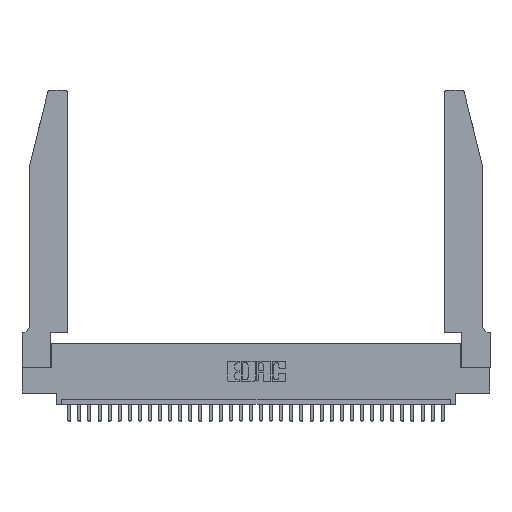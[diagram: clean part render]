
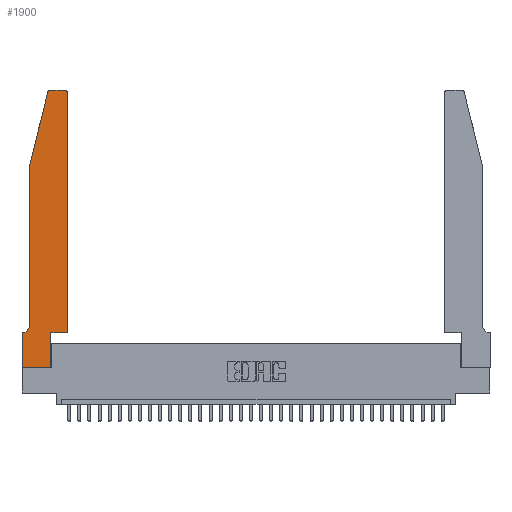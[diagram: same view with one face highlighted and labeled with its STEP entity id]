
A CAD part, top view. The second image highlights one B-rep face of the part: STEP entity #1900.
In plain terms, the highlighted planar face has unit normal (0, 0, 1).
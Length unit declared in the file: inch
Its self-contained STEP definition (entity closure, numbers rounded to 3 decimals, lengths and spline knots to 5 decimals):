
#378 = EDGE_CURVE ( 'NONE', #31666, #30595, #3601, .T. ) ;
#894 = CARTESIAN_POINT ( 'NONE',  ( 0.0055, 0.42, 0.37 ) ) ;
#1523 = VECTOR ( 'NONE', #24377, 39.37008 ) ;
#1820 = ORIENTED_EDGE ( 'NONE', *, *, #32897, .T. ) ;
#1900 = ADVANCED_FACE ( 'NONE', ( #3408 ), #12064, .T. ) ;
#1979 = CARTESIAN_POINT ( 'NONE',  ( 0.4205, 2.75, 0.37 ) ) ;
#1986 = LINE ( 'NONE', #2097, #11055 ) ;
#2097 = CARTESIAN_POINT ( 'NONE',  ( 0.2605, 2.75, 0.37 ) ) ;
#2234 = DIRECTION ( 'NONE',  ( 0., -1., 0. ) ) ;
#2243 = AXIS2_PLACEMENT_3D ( 'NONE', #894, #24611, #29582 ) ;
#2337 = VERTEX_POINT ( 'NONE', #3133 ) ;
#2358 = CARTESIAN_POINT ( 'NONE',  ( 0., 0.35, 0.37 ) ) ;
#2550 = DIRECTION ( 'NONE',  ( -1., 0., 0. ) ) ;
#2717 = ORIENTED_EDGE ( 'NONE', *, *, #17751, .T. ) ;
#3133 = CARTESIAN_POINT ( 'NONE',  ( 0.0755, 0.42, 0.37 ) ) ;
#3337 = CARTESIAN_POINT ( 'NONE',  ( 0.4505, 0.35, 0.37 ) ) ;
#3408 = FACE_OUTER_BOUND ( 'NONE', #11539, .T. ) ;
#3601 = LINE ( 'NONE', #29055, #6927 ) ;
#3641 = CARTESIAN_POINT ( 'NONE',  ( 0.0755, 2., 0.37 ) ) ;
#4012 = CARTESIAN_POINT ( 'NONE',  ( 0.284, 2.75, 0.37 ) ) ;
#4255 = CARTESIAN_POINT ( 'NONE',  ( 0.2865, 0., 0.37 ) ) ;
#4314 = DIRECTION ( 'NONE',  ( 0., 0., 1. ) ) ;
#4411 = CARTESIAN_POINT ( 'NONE',  ( 0., 0., 0.37 ) ) ;
#4863 = ORIENTED_EDGE ( 'NONE', *, *, #7968, .T. ) ;
#4931 = DIRECTION ( 'NONE',  ( 0., 1., 0. ) ) ;
#5988 = DIRECTION ( 'NONE',  ( 1., 0., 0. ) ) ;
#5998 = DIRECTION ( 'NONE',  ( 0., 1., 0. ) ) ;
#6377 = CIRCLE ( 'NONE', #2243, 0.07 ) ;
#6534 = EDGE_CURVE ( 'NONE', #27630, #6646, #17616, .T. ) ;
#6646 = VERTEX_POINT ( 'NONE', #3641 ) ;
#6927 = VECTOR ( 'NONE', #29381, 39.37008 ) ;
#6980 = ORIENTED_EDGE ( 'NONE', *, *, #10887, .T. ) ;
#7105 = VERTEX_POINT ( 'NONE', #20014 ) ;
#7160 = CARTESIAN_POINT ( 'NONE',  ( 0.25487, 2.72718, 0.37 ) ) ;
#7968 = EDGE_CURVE ( 'NONE', #30595, #17654, #28152, .T. ) ;
#8931 = LINE ( 'NONE', #17839, #16777 ) ;
#8942 = CIRCLE ( 'NONE', #20503, 0.03 ) ;
#9173 = EDGE_CURVE ( 'NONE', #28556, #18429, #1986, .T. ) ;
#9708 = VERTEX_POINT ( 'NONE', #11129 ) ;
#10887 = EDGE_CURVE ( 'NONE', #28252, #9708, #18419, .T. ) ;
#11055 = VECTOR ( 'NONE', #2550, 39.37008 ) ;
#11129 = CARTESIAN_POINT ( 'NONE',  ( 0.4505, 2.72, 0.37 ) ) ;
#11187 = CARTESIAN_POINT ( 'NONE',  ( 0., 0., 0.37 ) ) ;
#11539 = EDGE_LOOP ( 'NONE', ( #31238, #1820, #30203, #26848, #13171, #14129, #4863, #19136, #22132, #2717, #6980, #32469 ) ) ;
#11841 = VECTOR ( 'NONE', #16122, 39.37008 ) ;
#12064 = PLANE ( 'NONE',  #31644 ) ;
#12303 = DIRECTION ( 'NONE',  ( 0., -1., 0. ) ) ;
#13074 = VECTOR ( 'NONE', #4931, 39.37008 ) ;
#13120 = LINE ( 'NONE', #24601, #29118 ) ;
#13171 = ORIENTED_EDGE ( 'NONE', *, *, #31461, .T. ) ;
#14061 = CARTESIAN_POINT ( 'NONE',  ( 0.4205, 2.72, 0.37 ) ) ;
#14129 = ORIENTED_EDGE ( 'NONE', *, *, #378, .T. ) ;
#14179 = VECTOR ( 'NONE', #5998, 39.37008 ) ;
#14575 = LINE ( 'NONE', #26937, #14179 ) ;
#15140 = CARTESIAN_POINT ( 'NONE',  ( 0., 0., 0.37 ) ) ;
#15602 = VERTEX_POINT ( 'NONE', #4255 ) ;
#15848 = VECTOR ( 'NONE', #2234, 39.37008 ) ;
#16013 = DIRECTION ( 'NONE',  ( 0., 0., 1. ) ) ;
#16122 = DIRECTION ( 'NONE',  ( -0.239, -0.971, 0. ) ) ;
#16777 = VECTOR ( 'NONE', #12303, 39.37008 ) ;
#16804 = DIRECTION ( 'NONE',  ( 1., 0., 0. ) ) ;
#17616 = LINE ( 'NONE', #25666, #11841 ) ;
#17654 = VERTEX_POINT ( 'NONE', #15140 ) ;
#17751 = EDGE_CURVE ( 'NONE', #7105, #28252, #13120, .T. ) ;
#17775 = EDGE_CURVE ( 'NONE', #17654, #15602, #21283, .T. ) ;
#17839 = CARTESIAN_POINT ( 'NONE',  ( 0.0755, 2., 0.37 ) ) ;
#18261 = EDGE_CURVE ( 'NONE', #6646, #2337, #8931, .T. ) ;
#18419 = LINE ( 'NONE', #31295, #13074 ) ;
#18429 = VERTEX_POINT ( 'NONE', #4012 ) ;
#18443 = CARTESIAN_POINT ( 'NONE',  ( 0.284, 2.72, 0.37 ) ) ;
#19136 = ORIENTED_EDGE ( 'NONE', *, *, #17775, .T. ) ;
#19313 = DIRECTION ( 'NONE',  ( 0., 0., 1. ) ) ;
#20012 = EDGE_CURVE ( 'NONE', #15602, #7105, #14575, .T. ) ;
#20014 = CARTESIAN_POINT ( 'NONE',  ( 0.2865, 0.35, 0.37 ) ) ;
#20503 = AXIS2_PLACEMENT_3D ( 'NONE', #14061, #19313, #16804 ) ;
#21283 = LINE ( 'NONE', #11187, #1523 ) ;
#22132 = ORIENTED_EDGE ( 'NONE', *, *, #20012, .T. ) ;
#22739 = DIRECTION ( 'NONE',  ( 1., 0., 0. ) ) ;
#24377 = DIRECTION ( 'NONE',  ( 1., 0., 0. ) ) ;
#24601 = CARTESIAN_POINT ( 'NONE',  ( 0.4505, 0.35, 0.37 ) ) ;
#24611 = DIRECTION ( 'NONE',  ( 0., 0., -1. ) ) ;
#25666 = CARTESIAN_POINT ( 'NONE',  ( 0.0755, 2., 0.37 ) ) ;
#26848 = ORIENTED_EDGE ( 'NONE', *, *, #18261, .T. ) ;
#26937 = CARTESIAN_POINT ( 'NONE',  ( 0.2865, 0.35, 0.37 ) ) ;
#27630 = VERTEX_POINT ( 'NONE', #7160 ) ;
#28152 = LINE ( 'NONE', #4411, #15848 ) ;
#28252 = VERTEX_POINT ( 'NONE', #3337 ) ;
#28556 = VERTEX_POINT ( 'NONE', #1979 ) ;
#28569 = CIRCLE ( 'NONE', #29805, 0.03 ) ;
#29055 = CARTESIAN_POINT ( 'NONE',  ( 0.0755, 0.35, 0.37 ) ) ;
#29118 = VECTOR ( 'NONE', #5988, 39.37008 ) ;
#29381 = DIRECTION ( 'NONE',  ( -1., 0., 0. ) ) ;
#29582 = DIRECTION ( 'NONE',  ( -1., 0., 0. ) ) ;
#29805 = AXIS2_PLACEMENT_3D ( 'NONE', #18443, #16013, #31535 ) ;
#30203 = ORIENTED_EDGE ( 'NONE', *, *, #6534, .T. ) ;
#30220 = EDGE_CURVE ( 'NONE', #9708, #28556, #8942, .T. ) ;
#30577 = CARTESIAN_POINT ( 'NONE',  ( 0., 0.35, 0.37 ) ) ;
#30595 = VERTEX_POINT ( 'NONE', #2358 ) ;
#31238 = ORIENTED_EDGE ( 'NONE', *, *, #9173, .T. ) ;
#31295 = CARTESIAN_POINT ( 'NONE',  ( 0.4505, 0.35, 0.37 ) ) ;
#31461 = EDGE_CURVE ( 'NONE', #2337, #31666, #6377, .T. ) ;
#31535 = DIRECTION ( 'NONE',  ( 1., 0., 0. ) ) ;
#31644 = AXIS2_PLACEMENT_3D ( 'NONE', #30577, #4314, #22739 ) ;
#31666 = VERTEX_POINT ( 'NONE', #32006 ) ;
#32006 = CARTESIAN_POINT ( 'NONE',  ( 0.0055, 0.35, 0.37 ) ) ;
#32469 = ORIENTED_EDGE ( 'NONE', *, *, #30220, .T. ) ;
#32897 = EDGE_CURVE ( 'NONE', #18429, #27630, #28569, .T. ) ;
